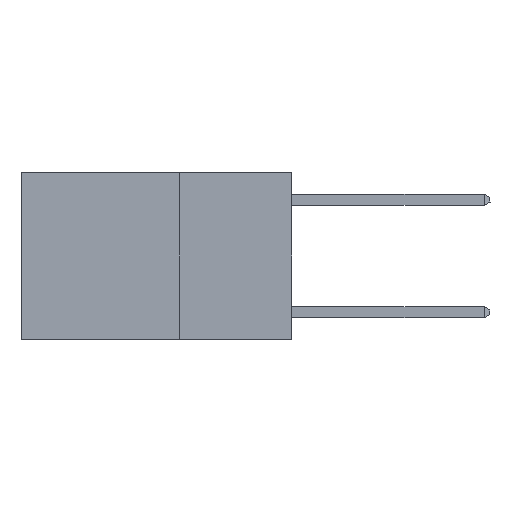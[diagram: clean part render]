
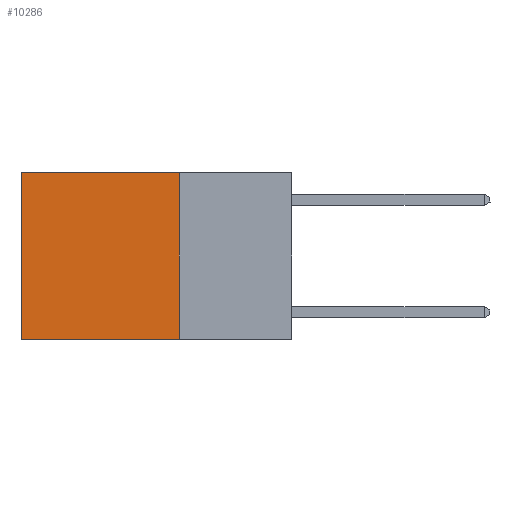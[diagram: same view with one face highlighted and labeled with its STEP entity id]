
A CAD part, left-side view. The second image highlights one B-rep face of the part: STEP entity #10286.
In plain terms, the highlighted planar face has unit normal (-1, 0, 0).
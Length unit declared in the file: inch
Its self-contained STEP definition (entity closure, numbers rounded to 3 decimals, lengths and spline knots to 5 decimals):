
#85 = VECTOR ( 'NONE', #8755, 39.37008 ) ;
#612 = FACE_OUTER_BOUND ( 'NONE', #1308, .T. ) ;
#796 = LINE ( 'NONE', #24045, #3776 ) ;
#1308 = EDGE_LOOP ( 'NONE', ( #3507, #16253, #12370, #14062 ) ) ;
#1354 = DIRECTION ( 'NONE',  ( 0., 0., -1. ) ) ;
#3507 = ORIENTED_EDGE ( 'NONE', *, *, #20637, .T. ) ;
#3776 = VECTOR ( 'NONE', #1354, 39.37008 ) ;
#3838 = CARTESIAN_POINT ( 'NONE',  ( 0.2625, 0.6, 0. ) ) ;
#4430 = CARTESIAN_POINT ( 'NONE',  ( 0.2625, 0.25, -0.37 ) ) ;
#4930 = LINE ( 'NONE', #9385, #17901 ) ;
#5221 = CARTESIAN_POINT ( 'NONE',  ( 0.2625, 0.25, 0. ) ) ;
#5925 = VERTEX_POINT ( 'NONE', #22262 ) ;
#6943 = PLANE ( 'NONE',  #16333 ) ;
#8383 = LINE ( 'NONE', #5221, #85 ) ;
#8755 = DIRECTION ( 'NONE',  ( 0., 1., 0. ) ) ;
#9385 = CARTESIAN_POINT ( 'NONE',  ( 0.2625, 0.25, -0.37 ) ) ;
#10286 = ADVANCED_FACE ( 'NONE', ( #612 ), #6943, .F. ) ;
#10582 = CARTESIAN_POINT ( 'NONE',  ( 0.2625, 0.6, 0. ) ) ;
#10736 = VERTEX_POINT ( 'NONE', #10582 ) ;
#11213 = EDGE_CURVE ( 'NONE', #5925, #10736, #8383, .T. ) ;
#12370 = ORIENTED_EDGE ( 'NONE', *, *, #21479, .F. ) ;
#12781 = CARTESIAN_POINT ( 'NONE',  ( 0.2625, 0.25, 0. ) ) ;
#14062 = ORIENTED_EDGE ( 'NONE', *, *, #11213, .T. ) ;
#14545 = VERTEX_POINT ( 'NONE', #20761 ) ;
#14670 = VERTEX_POINT ( 'NONE', #4430 ) ;
#16253 = ORIENTED_EDGE ( 'NONE', *, *, #16512, .F. ) ;
#16333 = AXIS2_PLACEMENT_3D ( 'NONE', #12781, #16584, #21966 ) ;
#16512 = EDGE_CURVE ( 'NONE', #14670, #14545, #4930, .T. ) ;
#16584 = DIRECTION ( 'NONE',  ( 1., 0., 0. ) ) ;
#17901 = VECTOR ( 'NONE', #20526, 39.37008 ) ;
#18254 = VECTOR ( 'NONE', #22499, 39.37008 ) ;
#19096 = LINE ( 'NONE', #3838, #18254 ) ;
#20526 = DIRECTION ( 'NONE',  ( 0., 1., 0. ) ) ;
#20637 = EDGE_CURVE ( 'NONE', #10736, #14545, #19096, .T. ) ;
#20761 = CARTESIAN_POINT ( 'NONE',  ( 0.2625, 0.6, -0.37 ) ) ;
#21479 = EDGE_CURVE ( 'NONE', #5925, #14670, #796, .T. ) ;
#21966 = DIRECTION ( 'NONE',  ( 0., 0., -1. ) ) ;
#22262 = CARTESIAN_POINT ( 'NONE',  ( 0.2625, 0.25, 0. ) ) ;
#22499 = DIRECTION ( 'NONE',  ( 0., 0., -1. ) ) ;
#24045 = CARTESIAN_POINT ( 'NONE',  ( 0.2625, 0.25, 0. ) ) ;
